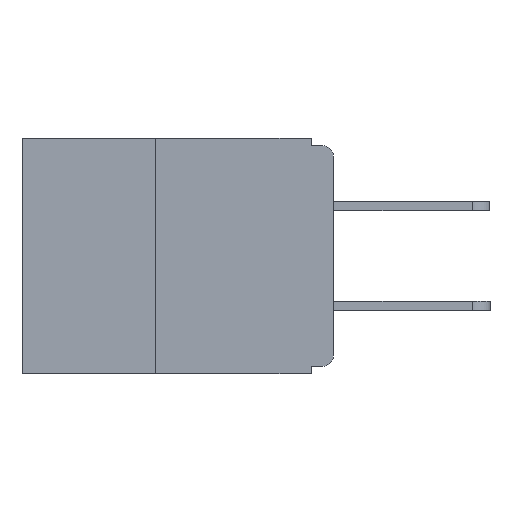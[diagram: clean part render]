
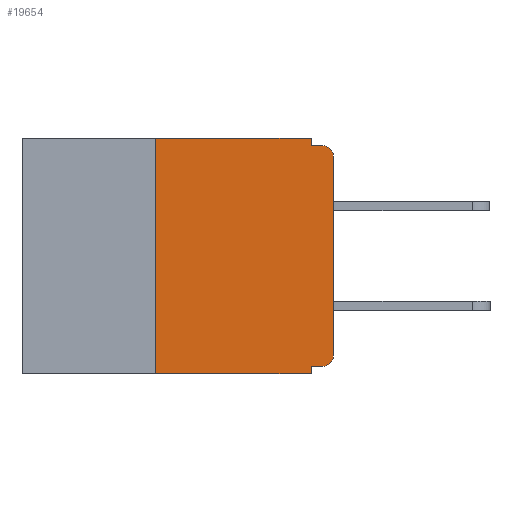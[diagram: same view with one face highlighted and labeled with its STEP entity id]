
A CAD part, left-side view. The second image highlights one B-rep face of the part: STEP entity #19654.
In plain terms, the highlighted planar face has unit normal (-1, 0, 0).
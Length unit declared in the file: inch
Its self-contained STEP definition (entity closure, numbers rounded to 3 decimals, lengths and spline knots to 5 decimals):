
#72 = EDGE_CURVE ( 'NONE', #483, #15872, #13637, .T. ) ;
#86 = DIRECTION ( 'NONE',  ( 0., 0., -1. ) ) ;
#149 = VERTEX_POINT ( 'NONE', #15505 ) ;
#483 = VERTEX_POINT ( 'NONE', #24577 ) ;
#853 = ORIENTED_EDGE ( 'NONE', *, *, #24663, .F. ) ;
#1233 = VERTEX_POINT ( 'NONE', #10537 ) ;
#1264 = CARTESIAN_POINT ( 'NONE',  ( 0., 0., 0. ) ) ;
#2245 = CARTESIAN_POINT ( 'NONE',  ( 0., 0.031, -0.33 ) ) ;
#2472 = LINE ( 'NONE', #14428, #28241 ) ;
#3012 = VECTOR ( 'NONE', #29945, 39.37008 ) ;
#3319 = EDGE_CURVE ( 'NONE', #27391, #29801, #6325, .T. ) ;
#3322 = VECTOR ( 'NONE', #5851, 39.37008 ) ;
#3323 = VERTEX_POINT ( 'NONE', #7361 ) ;
#3363 = CARTESIAN_POINT ( 'NONE',  ( 0., 0.437, 0. ) ) ;
#3810 = CARTESIAN_POINT ( 'NONE',  ( 0., 0., -0.01 ) ) ;
#5851 = DIRECTION ( 'NONE',  ( 0., -1., 0. ) ) ;
#6193 = ORIENTED_EDGE ( 'NONE', *, *, #9976, .F. ) ;
#6325 = CIRCLE ( 'NONE', #16663, 0.015 ) ;
#6709 = ORIENTED_EDGE ( 'NONE', *, *, #8215, .F. ) ;
#6726 = DIRECTION ( 'NONE',  ( 0., 0., -1. ) ) ;
#6853 = DIRECTION ( 'NONE',  ( -1., 0., 0. ) ) ;
#6950 = CARTESIAN_POINT ( 'NONE',  ( 0., 0.015, -0.025 ) ) ;
#7361 = CARTESIAN_POINT ( 'NONE',  ( 0., 0.031, 0. ) ) ;
#8075 = CARTESIAN_POINT ( 'NONE',  ( 0., 0., -0.305 ) ) ;
#8215 = EDGE_CURVE ( 'NONE', #483, #149, #8721, .T. ) ;
#8695 = DIRECTION ( 'NONE',  ( 0., 0., 1. ) ) ;
#8715 = DIRECTION ( 'NONE',  ( 0., -1., 0. ) ) ;
#8721 = LINE ( 'NONE', #11417, #3012 ) ;
#9693 = ORIENTED_EDGE ( 'NONE', *, *, #72, .T. ) ;
#9768 = LINE ( 'NONE', #3363, #3322 ) ;
#9976 = EDGE_CURVE ( 'NONE', #10458, #3323, #9768, .T. ) ;
#10276 = ORIENTED_EDGE ( 'NONE', *, *, #3319, .T. ) ;
#10281 = VECTOR ( 'NONE', #8715, 39.37008 ) ;
#10458 = VERTEX_POINT ( 'NONE', #16317 ) ;
#10537 = CARTESIAN_POINT ( 'NONE',  ( 0., 0.031, -0.01 ) ) ;
#11197 = VECTOR ( 'NONE', #17990, 39.37008 ) ;
#11417 = CARTESIAN_POINT ( 'NONE',  ( 0., 0., -0.32 ) ) ;
#11859 = ORIENTED_EDGE ( 'NONE', *, *, #19334, .F. ) ;
#13637 = CIRCLE ( 'NONE', #18377, 0.015 ) ;
#13995 = FACE_OUTER_BOUND ( 'NONE', #19952, .T. ) ;
#14104 = CARTESIAN_POINT ( 'NONE',  ( 0., 0.015, -0.01 ) ) ;
#14296 = CARTESIAN_POINT ( 'NONE',  ( 0., 0.437, -0.33 ) ) ;
#14428 = CARTESIAN_POINT ( 'NONE',  ( 0., 0.031, 0. ) ) ;
#14523 = DIRECTION ( 'NONE',  ( 1., 0., 0. ) ) ;
#14570 = ORIENTED_EDGE ( 'NONE', *, *, #18528, .F. ) ;
#15178 = ORIENTED_EDGE ( 'NONE', *, *, #30069, .T. ) ;
#15505 = CARTESIAN_POINT ( 'NONE',  ( 0., 0.031, -0.32 ) ) ;
#15872 = VERTEX_POINT ( 'NONE', #8075 ) ;
#16317 = CARTESIAN_POINT ( 'NONE',  ( 0., 0.25, 0. ) ) ;
#16663 = AXIS2_PLACEMENT_3D ( 'NONE', #6950, #6853, #6726 ) ;
#16735 = LINE ( 'NONE', #1264, #11197 ) ;
#17165 = VECTOR ( 'NONE', #8695, 39.37008 ) ;
#17805 = CARTESIAN_POINT ( 'NONE',  ( 0., 0.031, -0.33 ) ) ;
#17990 = DIRECTION ( 'NONE',  ( 0., 0., 1. ) ) ;
#18377 = AXIS2_PLACEMENT_3D ( 'NONE', #29213, #30296, #30207 ) ;
#18528 = EDGE_CURVE ( 'NONE', #149, #22795, #26716, .T. ) ;
#19076 = DIRECTION ( 'NONE',  ( 0., 0., -1. ) ) ;
#19166 = PLANE ( 'NONE',  #28090 ) ;
#19334 = EDGE_CURVE ( 'NONE', #1233, #29801, #22727, .T. ) ;
#19654 = ADVANCED_FACE ( 'NONE', ( #13995 ), #19166, .F. ) ;
#19952 = EDGE_LOOP ( 'NONE', ( #15178, #10276, #11859, #25869, #6193, #853, #20670, #14570, #6709, #9693 ) ) ;
#20659 = VECTOR ( 'NONE', #19076, 39.37008 ) ;
#20670 = ORIENTED_EDGE ( 'NONE', *, *, #23132, .T. ) ;
#21944 = VECTOR ( 'NONE', #28235, 39.37008 ) ;
#22595 = LINE ( 'NONE', #22736, #17165 ) ;
#22727 = LINE ( 'NONE', #3810, #10281 ) ;
#22736 = CARTESIAN_POINT ( 'NONE',  ( 0., 0.25, -0.33 ) ) ;
#22795 = VERTEX_POINT ( 'NONE', #17805 ) ;
#23132 = EDGE_CURVE ( 'NONE', #24915, #22795, #28043, .T. ) ;
#24577 = CARTESIAN_POINT ( 'NONE',  ( 0., 0.015, -0.32 ) ) ;
#24663 = EDGE_CURVE ( 'NONE', #24915, #10458, #22595, .T. ) ;
#24915 = VERTEX_POINT ( 'NONE', #26293 ) ;
#25869 = ORIENTED_EDGE ( 'NONE', *, *, #26193, .F. ) ;
#26193 = EDGE_CURVE ( 'NONE', #3323, #1233, #2472, .T. ) ;
#26293 = CARTESIAN_POINT ( 'NONE',  ( 0., 0.25, -0.33 ) ) ;
#26716 = LINE ( 'NONE', #2245, #20659 ) ;
#27391 = VERTEX_POINT ( 'NONE', #28399 ) ;
#28043 = LINE ( 'NONE', #14296, #21944 ) ;
#28090 = AXIS2_PLACEMENT_3D ( 'NONE', #28357, #14523, #86 ) ;
#28235 = DIRECTION ( 'NONE',  ( 0., -1., 0. ) ) ;
#28241 = VECTOR ( 'NONE', #28266, 39.37008 ) ;
#28266 = DIRECTION ( 'NONE',  ( 0., 0., -1. ) ) ;
#28357 = CARTESIAN_POINT ( 'NONE',  ( 0., 0.437, 0. ) ) ;
#28399 = CARTESIAN_POINT ( 'NONE',  ( 0., 0., -0.025 ) ) ;
#29213 = CARTESIAN_POINT ( 'NONE',  ( 0., 0.015, -0.305 ) ) ;
#29801 = VERTEX_POINT ( 'NONE', #14104 ) ;
#29945 = DIRECTION ( 'NONE',  ( 0., 1., 0. ) ) ;
#30069 = EDGE_CURVE ( 'NONE', #15872, #27391, #16735, .T. ) ;
#30207 = DIRECTION ( 'NONE',  ( 0., 0., -1. ) ) ;
#30296 = DIRECTION ( 'NONE',  ( -1., 0., 0. ) ) ;
